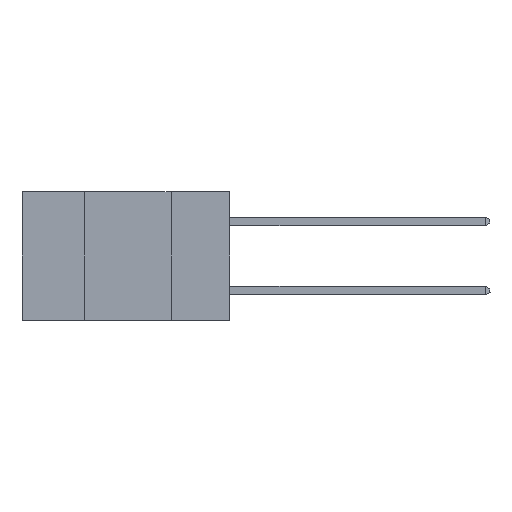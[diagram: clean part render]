
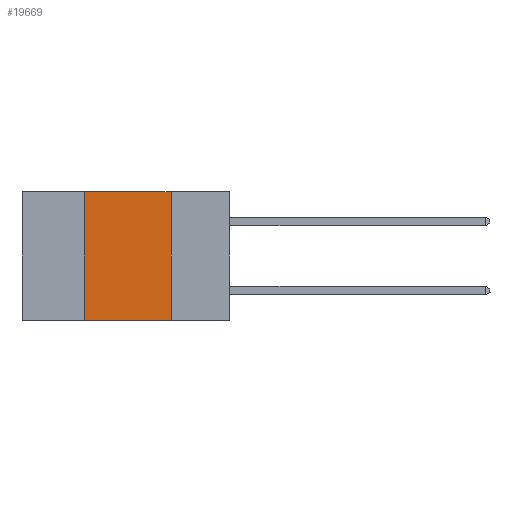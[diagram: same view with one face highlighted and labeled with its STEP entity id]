
A CAD part, left-side view. The second image highlights one B-rep face of the part: STEP entity #19669.
In plain terms, the highlighted planar face has unit normal (-1, 0, 0).
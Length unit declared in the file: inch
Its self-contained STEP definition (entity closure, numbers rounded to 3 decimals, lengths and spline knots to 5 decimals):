
#507 = DIRECTION ( 'NONE',  ( 0., 0., -1. ) ) ;
#906 = CARTESIAN_POINT ( 'NONE',  ( 0., 0.42, -0.37 ) ) ;
#1321 = DIRECTION ( 'NONE',  ( 0., 0., -1. ) ) ;
#1446 = CARTESIAN_POINT ( 'NONE',  ( 0., 0.6, -0.37 ) ) ;
#1730 = LINE ( 'NONE', #23337, #12729 ) ;
#2223 = CARTESIAN_POINT ( 'NONE',  ( 0., 0.42, 0. ) ) ;
#3589 = DIRECTION ( 'NONE',  ( 1., 0., 0. ) ) ;
#7358 = CARTESIAN_POINT ( 'NONE',  ( 0., 0.17, -0.37 ) ) ;
#10356 = VERTEX_POINT ( 'NONE', #11655 ) ;
#10782 = DIRECTION ( 'NONE',  ( 0., -1., 0. ) ) ;
#11018 = ORIENTED_EDGE ( 'NONE', *, *, #17891, .F. ) ;
#11237 = LINE ( 'NONE', #12457, #19111 ) ;
#11655 = CARTESIAN_POINT ( 'NONE',  ( 0., 0.17, 0. ) ) ;
#11978 = DIRECTION ( 'NONE',  ( 0., -1., 0. ) ) ;
#12457 = CARTESIAN_POINT ( 'NONE',  ( 0., 0.6, 0. ) ) ;
#12729 = VECTOR ( 'NONE', #17298, 39.37008 ) ;
#12804 = LINE ( 'NONE', #1446, #21644 ) ;
#13065 = LINE ( 'NONE', #24530, #18731 ) ;
#13504 = CARTESIAN_POINT ( 'NONE',  ( 0., 0.6, 0. ) ) ;
#14292 = AXIS2_PLACEMENT_3D ( 'NONE', #13504, #3589, #1321 ) ;
#14474 = PLANE ( 'NONE',  #14292 ) ;
#15561 = VERTEX_POINT ( 'NONE', #906 ) ;
#16144 = EDGE_CURVE ( 'NONE', #15561, #16389, #1730, .T. ) ;
#16389 = VERTEX_POINT ( 'NONE', #2223 ) ;
#17298 = DIRECTION ( 'NONE',  ( 0., 0., 1. ) ) ;
#17891 = EDGE_CURVE ( 'NONE', #16389, #10356, #11237, .T. ) ;
#18622 = EDGE_CURVE ( 'NONE', #10356, #22801, #13065, .T. ) ;
#18731 = VECTOR ( 'NONE', #507, 39.37008 ) ;
#18906 = ORIENTED_EDGE ( 'NONE', *, *, #23478, .T. ) ;
#19111 = VECTOR ( 'NONE', #10782, 39.37008 ) ;
#19669 = ADVANCED_FACE ( 'NONE', ( #19970 ), #14474, .F. ) ;
#19970 = FACE_OUTER_BOUND ( 'NONE', #21627, .T. ) ;
#21627 = EDGE_LOOP ( 'NONE', ( #23234, #11018, #25270, #18906 ) ) ;
#21644 = VECTOR ( 'NONE', #11978, 39.37008 ) ;
#22801 = VERTEX_POINT ( 'NONE', #7358 ) ;
#23234 = ORIENTED_EDGE ( 'NONE', *, *, #18622, .F. ) ;
#23337 = CARTESIAN_POINT ( 'NONE',  ( 0., 0.42, 0. ) ) ;
#23478 = EDGE_CURVE ( 'NONE', #15561, #22801, #12804, .T. ) ;
#24530 = CARTESIAN_POINT ( 'NONE',  ( 0., 0.17, 0. ) ) ;
#25270 = ORIENTED_EDGE ( 'NONE', *, *, #16144, .F. ) ;
